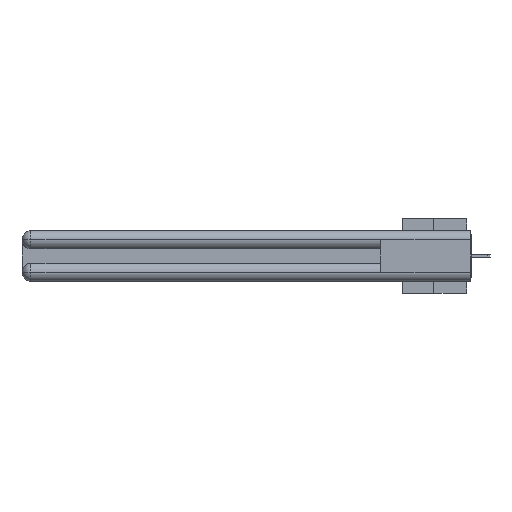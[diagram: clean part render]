
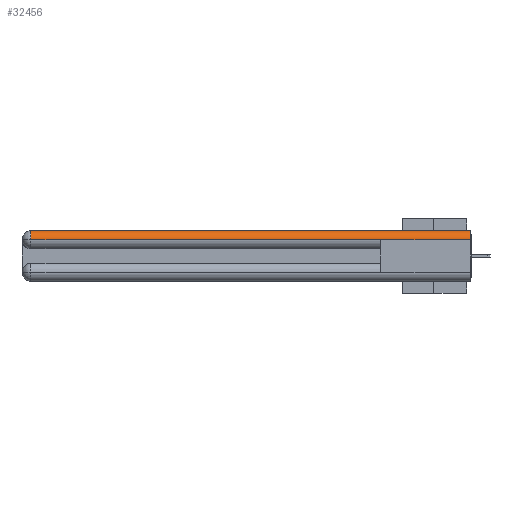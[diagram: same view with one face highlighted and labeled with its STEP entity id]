
A CAD part, left-side view. The second image highlights one B-rep face of the part: STEP entity #32456.
In plain terms, the highlighted cylindrical face has radius 1.562 mm (diameter 3.124 mm), a partial arc.
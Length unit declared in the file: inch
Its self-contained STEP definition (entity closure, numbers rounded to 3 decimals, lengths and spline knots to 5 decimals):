
#153 = ORIENTED_EDGE ( 'NONE', *, *, #40346, .F. ) ;
#1834 = EDGE_CURVE ( 'NONE', #16837, #26928, #4772, .T. ) ;
#3224 = CARTESIAN_POINT ( 'NONE',  ( 0., 2.94, -0.0615 ) ) ;
#3256 = LINE ( 'NONE', #39441, #22557 ) ;
#3604 = CARTESIAN_POINT ( 'NONE',  ( 0., 0.6, -0.0615 ) ) ;
#3605 = DIRECTION ( 'NONE',  ( 0., -1., 0. ) ) ;
#4772 = CIRCLE ( 'NONE', #8211, 0.0615 ) ;
#5922 = DIRECTION ( 'NONE',  ( 0., 1., 0. ) ) ;
#8211 = AXIS2_PLACEMENT_3D ( 'NONE', #13998, #30190, #40067 ) ;
#9273 = ORIENTED_EDGE ( 'NONE', *, *, #23736, .F. ) ;
#11704 = DIRECTION ( 'NONE',  ( 0., 0., 1. ) ) ;
#12006 = EDGE_CURVE ( 'NONE', #37059, #26651, #30531, .T. ) ;
#13692 = AXIS2_PLACEMENT_3D ( 'NONE', #25342, #5922, #21687 ) ;
#13857 = DIRECTION ( 'NONE',  ( 0., -1., 0. ) ) ;
#13998 = CARTESIAN_POINT ( 'NONE',  ( 0.0615, 0., -0.0615 ) ) ;
#14931 = CARTESIAN_POINT ( 'NONE',  ( 0.0615, 2.94, -0.0615 ) ) ;
#15613 = CYLINDRICAL_SURFACE ( 'NONE', #13692, 0.0615 ) ;
#15664 = ORIENTED_EDGE ( 'NONE', *, *, #1834, .F. ) ;
#16837 = VERTEX_POINT ( 'NONE', #41505 ) ;
#19309 = ORIENTED_EDGE ( 'NONE', *, *, #42378, .T. ) ;
#21548 = VECTOR ( 'NONE', #13857, 39.37008 ) ;
#21687 = DIRECTION ( 'NONE',  ( 0., 0., 1. ) ) ;
#22450 = DIRECTION ( 'NONE',  ( 0., 1., 0. ) ) ;
#22557 = VECTOR ( 'NONE', #22450, 39.37008 ) ;
#23736 = EDGE_CURVE ( 'NONE', #26928, #31013, #3256, .T. ) ;
#24314 = AXIS2_PLACEMENT_3D ( 'NONE', #14931, #34561, #11704 ) ;
#25342 = CARTESIAN_POINT ( 'NONE',  ( 0.0615, 0., -0.0615 ) ) ;
#26651 = VERTEX_POINT ( 'NONE', #3224 ) ;
#26928 = VERTEX_POINT ( 'NONE', #39596 ) ;
#28156 = FACE_OUTER_BOUND ( 'NONE', #29289, .T. ) ;
#29289 = EDGE_LOOP ( 'NONE', ( #153, #37460, #19309, #9273, #15664 ) ) ;
#30190 = DIRECTION ( 'NONE',  ( 0., -1., 0. ) ) ;
#30531 = CIRCLE ( 'NONE', #24314, 0.0615 ) ;
#31013 = VERTEX_POINT ( 'NONE', #3604 ) ;
#32456 = ADVANCED_FACE ( 'NONE', ( #28156 ), #15613, .T. ) ;
#33121 = LINE ( 'NONE', #36125, #35417 ) ;
#34561 = DIRECTION ( 'NONE',  ( 0., -1., 0. ) ) ;
#34692 = CARTESIAN_POINT ( 'NONE',  ( 0.0615, 0., 0. ) ) ;
#35417 = VECTOR ( 'NONE', #3605, 39.37008 ) ;
#36125 = CARTESIAN_POINT ( 'NONE',  ( 0., 3., -0.0615 ) ) ;
#37059 = VERTEX_POINT ( 'NONE', #40976 ) ;
#37460 = ORIENTED_EDGE ( 'NONE', *, *, #12006, .T. ) ;
#37914 = LINE ( 'NONE', #34692, #21548 ) ;
#39441 = CARTESIAN_POINT ( 'NONE',  ( 0., 3., -0.0615 ) ) ;
#39596 = CARTESIAN_POINT ( 'NONE',  ( 0., 0., -0.0615 ) ) ;
#40067 = DIRECTION ( 'NONE',  ( 1., 0., 0. ) ) ;
#40346 = EDGE_CURVE ( 'NONE', #37059, #16837, #37914, .T. ) ;
#40976 = CARTESIAN_POINT ( 'NONE',  ( 0.0615, 2.94, 0. ) ) ;
#41505 = CARTESIAN_POINT ( 'NONE',  ( 0.0615, 0., 0. ) ) ;
#42378 = EDGE_CURVE ( 'NONE', #26651, #31013, #33121, .T. ) ;
